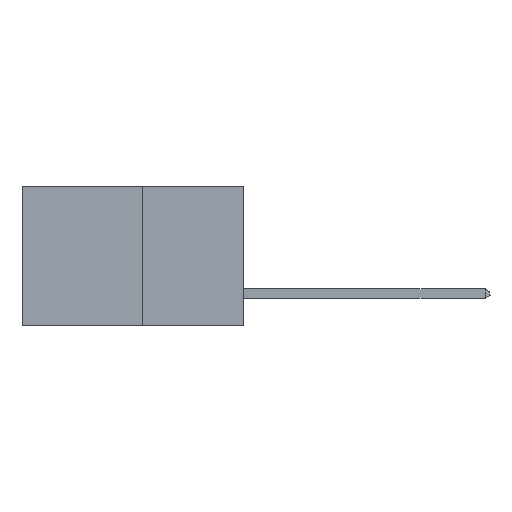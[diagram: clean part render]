
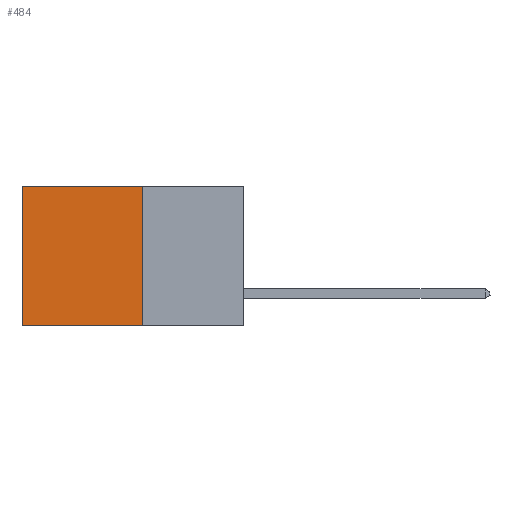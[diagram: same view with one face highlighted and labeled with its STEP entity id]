
A CAD part, left-side view. The second image highlights one B-rep face of the part: STEP entity #484.
In plain terms, the highlighted planar face has unit normal (-1, 0, 0).
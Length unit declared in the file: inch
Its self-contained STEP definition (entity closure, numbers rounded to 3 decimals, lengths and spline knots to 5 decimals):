
#484 = ADVANCED_FACE ( 'NONE', ( #14303 ), #9624, .F. ) ;
#667 = CARTESIAN_POINT ( 'NONE',  ( 0.277, 0.59, -0.37 ) ) ;
#804 = VECTOR ( 'NONE', #4511, 39.37008 ) ;
#1234 = DIRECTION ( 'NONE',  ( 0., 0., -1. ) ) ;
#1894 = EDGE_CURVE ( 'NONE', #5177, #15566, #13841, .T. ) ;
#1952 = EDGE_CURVE ( 'NONE', #10028, #15566, #5834, .T. ) ;
#3039 = VECTOR ( 'NONE', #11798, 39.37008 ) ;
#4010 = CARTESIAN_POINT ( 'NONE',  ( 0.277, 0.27, -0.37 ) ) ;
#4511 = DIRECTION ( 'NONE',  ( 0., 1., 0. ) ) ;
#5177 = VERTEX_POINT ( 'NONE', #8725 ) ;
#5211 = CARTESIAN_POINT ( 'NONE',  ( 0.277, 0.59, -0.37 ) ) ;
#5834 = LINE ( 'NONE', #9673, #12609 ) ;
#6328 = LINE ( 'NONE', #4010, #9992 ) ;
#8477 = EDGE_CURVE ( 'NONE', #14443, #10028, #6328, .T. ) ;
#8725 = CARTESIAN_POINT ( 'NONE',  ( 0.277, 0.59, 0. ) ) ;
#9512 = CARTESIAN_POINT ( 'NONE',  ( 0.277, 0.27, 0. ) ) ;
#9541 = DIRECTION ( 'NONE',  ( 1., 0., 0. ) ) ;
#9624 = PLANE ( 'NONE',  #9842 ) ;
#9673 = CARTESIAN_POINT ( 'NONE',  ( 0.277, 0.27, -0.37 ) ) ;
#9764 = DIRECTION ( 'NONE',  ( 0., 0., -1. ) ) ;
#9842 = AXIS2_PLACEMENT_3D ( 'NONE', #10034, #9541, #9764 ) ;
#9871 = ORIENTED_EDGE ( 'NONE', *, *, #8477, .F. ) ;
#9930 = CARTESIAN_POINT ( 'NONE',  ( 0.277, 0.27, -0.37 ) ) ;
#9992 = VECTOR ( 'NONE', #1234, 39.37008 ) ;
#10028 = VERTEX_POINT ( 'NONE', #9930 ) ;
#10034 = CARTESIAN_POINT ( 'NONE',  ( 0.277, 0.27, -0.37 ) ) ;
#10281 = DIRECTION ( 'NONE',  ( 0., 1., 0. ) ) ;
#10468 = ORIENTED_EDGE ( 'NONE', *, *, #1952, .F. ) ;
#11340 = CARTESIAN_POINT ( 'NONE',  ( 0.277, 0.27, 0. ) ) ;
#11355 = LINE ( 'NONE', #11340, #804 ) ;
#11533 = ORIENTED_EDGE ( 'NONE', *, *, #1894, .T. ) ;
#11771 = EDGE_LOOP ( 'NONE', ( #11533, #10468, #9871, #16671 ) ) ;
#11798 = DIRECTION ( 'NONE',  ( 0., 0., -1. ) ) ;
#12609 = VECTOR ( 'NONE', #10281, 39.37008 ) ;
#13841 = LINE ( 'NONE', #667, #3039 ) ;
#14303 = FACE_OUTER_BOUND ( 'NONE', #11771, .T. ) ;
#14443 = VERTEX_POINT ( 'NONE', #9512 ) ;
#14646 = EDGE_CURVE ( 'NONE', #14443, #5177, #11355, .T. ) ;
#15566 = VERTEX_POINT ( 'NONE', #5211 ) ;
#16671 = ORIENTED_EDGE ( 'NONE', *, *, #14646, .T. ) ;
